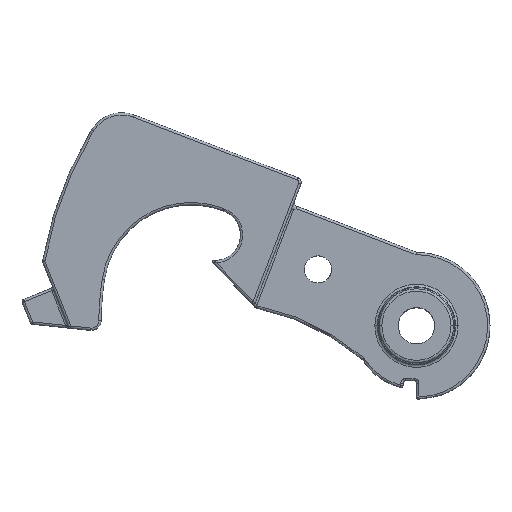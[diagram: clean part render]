
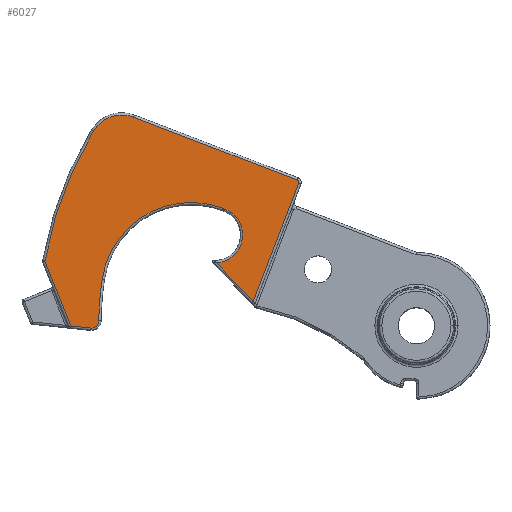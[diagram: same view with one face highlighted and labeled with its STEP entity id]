
A CAD part, top view. The second image highlights one B-rep face of the part: STEP entity #6027.
In plain terms, the highlighted planar face has unit normal (0, 0, 1).
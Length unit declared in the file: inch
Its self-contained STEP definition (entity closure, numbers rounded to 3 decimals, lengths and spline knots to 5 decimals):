
#661=CARTESIAN_POINT('',(-0.85704,0.26974,0.3));
#1833=DIRECTION('',(0.371,-0.929,0.));
#1834=VECTOR('',#1833,0.29883);
#1835=CARTESIAN_POINT('',(-1.59102,0.27729,0.3));
#1836=LINE('',#1835,#1834);
#1840=CARTESIAN_POINT('',(0.,0.,0.3));
#1841=DIRECTION('',(0.,0.,1.));
#1842=DIRECTION('',(-0.856,0.517,0.));
#1843=AXIS2_PLACEMENT_3D('',#1840,#1841,#1842);
#1848=CARTESIAN_POINT('',(-1.26187,0.76181,0.3));
#1849=DIRECTION('',(0.,0.,1.));
#1850=DIRECTION('',(0.358,0.934,0.));
#1851=AXIS2_PLACEMENT_3D('',#1848,#1849,#1850);
#1856=DIRECTION('',(-0.934,0.358,0.));
#1857=VECTOR('',#1856,0.75107);
#1858=CARTESIAN_POINT('',(-0.51016,0.62429,0.3));
#1859=LINE('',#1858,#1857);
#1863=CARTESIAN_POINT('',(-0.51374,0.61495,0.3));
#1864=DIRECTION('',(0.,0.,1.));
#1865=DIRECTION('',(0.934,-0.358,0.));
#1866=AXIS2_PLACEMENT_3D('',#1863,#1864,#1865);
#1871=DIRECTION('',(0.358,0.934,0.));
#1872=VECTOR('',#1871,0.54394);
#1873=CARTESIAN_POINT('',(-0.69934,0.10356,0.3));
#1874=LINE('',#1873,#1872);
#1878=DIRECTION('',(0.688,-0.725,0.));
#1879=VECTOR('',#1878,0.2291);
#1880=CARTESIAN_POINT('',(-0.85704,0.26974,0.3));
#1881=LINE('',#1880,#1879);
#1885=CARTESIAN_POINT('',(-0.86347,0.38892,0.3));
#1886=DIRECTION('',(0.,0.,-1.));
#1887=DIRECTION('',(1.,0.,0.));
#1888=AXIS2_PLACEMENT_3D('',#1885,#1886,#1887);
#1893=CARTESIAN_POINT('',(-0.86347,0.38892,0.3));
#1894=DIRECTION('',(0.,0.,-1.));
#1895=DIRECTION('',(0.358,0.934,0.));
#1896=AXIS2_PLACEMENT_3D('',#1893,#1894,#1895);
#1901=DIRECTION('',(0.934,-0.358,0.));
#1902=VECTOR('',#1901,0.00675);
#1903=CARTESIAN_POINT('',(-0.827,0.50276,0.3));
#1904=LINE('',#1903,#1902);
#1908=CARTESIAN_POINT('',(-0.96497,0.14334,0.3));
#1909=DIRECTION('',(0.,0.,-1.));
#1910=DIRECTION('',(-0.989,0.146,0.));
#1911=AXIS2_PLACEMENT_3D('',#1908,#1909,#1910);
#1916=CARTESIAN_POINT('',(0.,0.,0.3));
#1917=DIRECTION('',(0.,0.,-1.));
#1918=DIRECTION('',(-1.,0.015,0.));
#1919=AXIS2_PLACEMENT_3D('',#1916,#1917,#1918);
#1924=CARTESIAN_POINT('',(-1.39139,0.02156,0.3));
#1925=DIRECTION('',(0.,0.,1.));
#1926=DIRECTION('',(-0.105,-0.995,0.));
#1927=AXIS2_PLACEMENT_3D('',#1924,#1925,#1926);
#1932=DIRECTION('',(0.995,-0.105,0.));
#1933=VECTOR('',#1932,0.08612);
#1934=CARTESIAN_POINT('',(-1.48028,-0.00027,0.3));
#1935=LINE('',#1934,#1933);
#3972=CARTESIAN_POINT('',(-0.69934,0.10356,0.3));
#3973=VERTEX_POINT('',#3972);
#4024=CARTESIAN_POINT('',(-0.50441,0.61137,0.3));
#4026=VERTEX_POINT('',#4024);
#4187=CARTESIAN_POINT('',(-1.48028,-0.00027,0.3));
#4188=VERTEX_POINT('',#4187);
#4203=CARTESIAN_POINT('',(-1.39463,-0.00927,0.3));
#4204=VERTEX_POINT('',#4203);
#4308=CARTESIAN_POINT('',(-0.51016,0.62429,0.3));
#4309=VERTEX_POINT('',#4308);
#4418=VERTEX_POINT('',#661);
#4420=CARTESIAN_POINT('',(-1.3604,0.02108,0.3));
#4421=VERTEX_POINT('',#4420);
#4422=CARTESIAN_POINT('',(-1.34582,0.19973,0.3));
#4423=VERTEX_POINT('',#4422);
#4426=CARTESIAN_POINT('',(-0.827,0.50276,0.3));
#4427=VERTEX_POINT('',#4426);
#4430=CARTESIAN_POINT('',(-0.8207,0.50034,0.3));
#4431=VERTEX_POINT('',#4430);
#4432=CARTESIAN_POINT('',(-0.74411,0.38892,0.3));
#4433=VERTEX_POINT('',#4432);
#4446=CARTESIAN_POINT('',(-1.59102,0.27729,0.3));
#4448=VERTEX_POINT('',#4446);
#4458=CARTESIAN_POINT('',(-1.21134,0.89345,0.3));
#4459=VERTEX_POINT('',#4458);
#4460=CARTESIAN_POINT('',(-1.38258,0.83469,0.3));
#4462=VERTEX_POINT('',#4460);
#5995=CARTESIAN_POINT('',(-0.75349,0.30363,0.3));
#5996=DIRECTION('',(0.,0.,1.));
#5997=DIRECTION('',(1.,0.,0.));
#5998=AXIS2_PLACEMENT_3D('',#5995,#5996,#5997);
#5999=PLANE('',#5998);
#6000=ORIENTED_EDGE('',*,*,#5979,.F.);
#6002=ORIENTED_EDGE('',*,*,#6001,.F.);
#6004=ORIENTED_EDGE('',*,*,#6003,.F.);
#6006=ORIENTED_EDGE('',*,*,#6005,.F.);
#6008=ORIENTED_EDGE('',*,*,#6007,.F.);
#6009=ORIENTED_EDGE('',*,*,#5013,.F.);
#6010=ORIENTED_EDGE('',*,*,#5051,.F.);
#6012=ORIENTED_EDGE('',*,*,#6011,.F.);
#6014=ORIENTED_EDGE('',*,*,#6013,.F.);
#6016=ORIENTED_EDGE('',*,*,#6015,.F.);
#6018=ORIENTED_EDGE('',*,*,#6017,.F.);
#6020=ORIENTED_EDGE('',*,*,#6019,.F.);
#6022=ORIENTED_EDGE('',*,*,#6021,.F.);
#6024=ORIENTED_EDGE('',*,*,#6023,.F.);
#6025=EDGE_LOOP('',(#6000,#6002,#6004,#6006,#6008,#6009,#6010,#6012,#6014,#6016,
#6018,#6020,#6022,#6024));
#6026=FACE_OUTER_BOUND('',#6025,.F.);
#1844=CIRCLE('',#1843,1.615);
#1852=CIRCLE('',#1851,0.141);
#1867=CIRCLE('',#1866,0.01);
#1889=CIRCLE('',#1888,0.11935);
#1897=CIRCLE('',#1896,0.11935);
#1912=CIRCLE('',#1911,0.385);
#1920=CIRCLE('',#1919,1.36056);
#1928=CIRCLE('',#1927,0.031);
#5013=EDGE_CURVE('',#3973,#4026,#1874,.T.);
#5051=EDGE_CURVE('',#4418,#3973,#1881,.T.);
#5979=EDGE_CURVE('',#4448,#4188,#1836,.T.);
#6001=EDGE_CURVE('',#4462,#4448,#1844,.T.);
#6003=EDGE_CURVE('',#4459,#4462,#1852,.T.);
#6005=EDGE_CURVE('',#4309,#4459,#1859,.T.);
#6007=EDGE_CURVE('',#4026,#4309,#1867,.T.);
#6011=EDGE_CURVE('',#4433,#4418,#1889,.T.);
#6013=EDGE_CURVE('',#4431,#4433,#1897,.T.);
#6015=EDGE_CURVE('',#4427,#4431,#1904,.T.);
#6017=EDGE_CURVE('',#4423,#4427,#1912,.T.);
#6019=EDGE_CURVE('',#4421,#4423,#1920,.T.);
#6021=EDGE_CURVE('',#4204,#4421,#1928,.T.);
#6023=EDGE_CURVE('',#4188,#4204,#1935,.T.);
#6027=ADVANCED_FACE('',(#6026),#5999,.T.);
